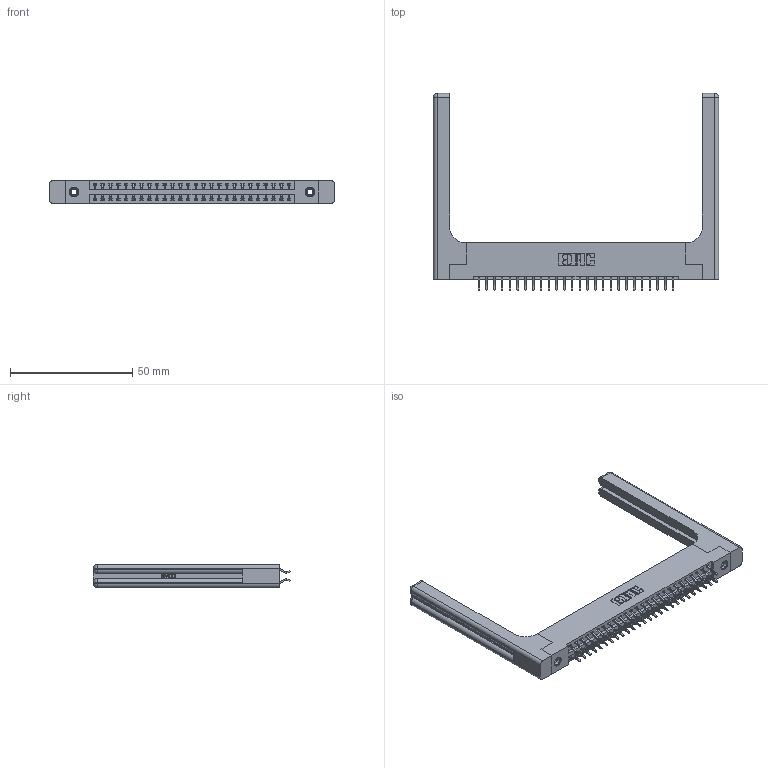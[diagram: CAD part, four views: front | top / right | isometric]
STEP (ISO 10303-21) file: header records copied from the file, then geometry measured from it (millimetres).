
FILE_DESCRIPTION (( 'STEP AP203' ), '1' );
FILE_NAME ('346-052-556-258.STEP', '2022-05-21T01:48:28', ( '' ), ( '' ), 'SwSTEP 2.0', 'SolidWorks 2020', '' );
FILE_SCHEMA (( 'CONFIG_CONTROL_DESIGN' ));
Length unit declared in the file: inch
Products named in the file (5): 345-292-001_556 Tail; 346 Part_Flush Mounting Lugs - 0.156 Dia-TH; 345-250-001_345-250-001-102; 346-220-058_345-220-058; 346-052-556-258
Assembly tree (57 placements, depth 2):
  346-052-556-258
    346 Part_Flush Mounting Lugs - 0.156 Dia-TH
    345-292-001_556 Tail  x52
    345-250-001_345-250-001-102  x2
    346-220-058_345-220-058  x2
Bounding box: 116.61 x 80.53 x 9.4 mm (x, y, z)
Volume: 18720.9 mm3; surface area: 20139.3 mm2
Topology: 57 solids, 57 shells, 3408 faces, 10027 edges, 6594 vertices
Faces by surface type: plane 2266, cylinder 1082, bspline 36, cone 12, sphere 8, torus 4
Entity records: 24940 total; most frequent: CARTESIAN_POINT 5159, ORIENTED_EDGE 3876, DIRECTION 3518, EDGE_CURVE 1938, VECTOR 1602, LINE 1602, VERTEX_POINT 1282, AXIS2_PLACEMENT_3D 958
